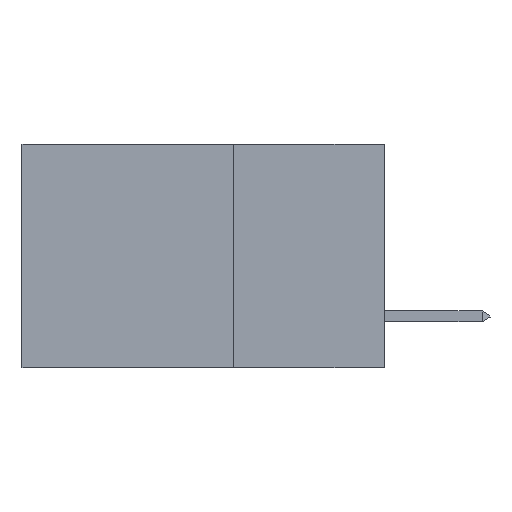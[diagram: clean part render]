
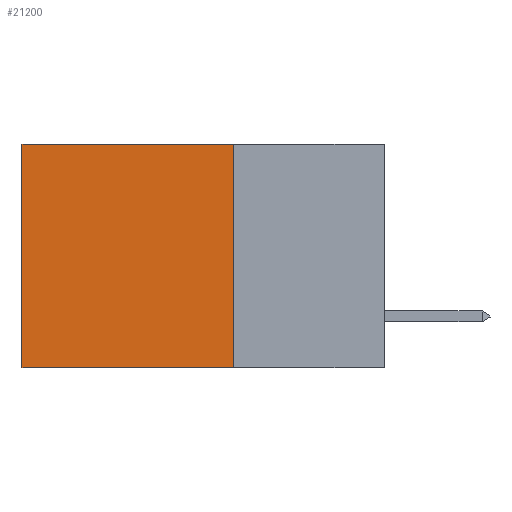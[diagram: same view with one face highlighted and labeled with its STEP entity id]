
A CAD part, left-side view. The second image highlights one B-rep face of the part: STEP entity #21200.
In plain terms, the highlighted planar face has unit normal (-1, 0, 0).
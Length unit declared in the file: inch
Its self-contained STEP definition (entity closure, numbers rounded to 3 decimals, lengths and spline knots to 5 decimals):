
#949 = FACE_OUTER_BOUND ( 'NONE', #18222, .T. ) ;
#1046 = VERTEX_POINT ( 'NONE', #7739 ) ;
#1164 = AXIS2_PLACEMENT_3D ( 'NONE', #21474, #10607, #21871 ) ;
#1707 = DIRECTION ( 'NONE',  ( 0., 0., -1. ) ) ;
#2795 = DIRECTION ( 'NONE',  ( 0., 1., 0. ) ) ;
#3478 = DIRECTION ( 'NONE',  ( 0., 1., 0. ) ) ;
#4974 = EDGE_CURVE ( 'NONE', #7376, #13451, #21937, .T. ) ;
#6647 = CARTESIAN_POINT ( 'NONE',  ( 0.2875, 0.6, 0. ) ) ;
#6938 = CARTESIAN_POINT ( 'NONE',  ( 0.2875, 0.25, -0.37 ) ) ;
#7376 = VERTEX_POINT ( 'NONE', #16361 ) ;
#7659 = LINE ( 'NONE', #6938, #8330 ) ;
#7739 = CARTESIAN_POINT ( 'NONE',  ( 0.2875, 0.6, -0.37 ) ) ;
#8107 = DIRECTION ( 'NONE',  ( 0., 0., -1. ) ) ;
#8330 = VECTOR ( 'NONE', #2795, 39.37008 ) ;
#8771 = VECTOR ( 'NONE', #3478, 39.37008 ) ;
#10059 = EDGE_CURVE ( 'NONE', #13451, #1046, #14945, .T. ) ;
#10607 = DIRECTION ( 'NONE',  ( 1., 0., 0. ) ) ;
#10647 = EDGE_CURVE ( 'NONE', #7376, #24971, #27778, .T. ) ;
#11084 = ORIENTED_EDGE ( 'NONE', *, *, #10647, .F. ) ;
#12670 = CARTESIAN_POINT ( 'NONE',  ( 0.2875, 0.6, 0. ) ) ;
#13451 = VERTEX_POINT ( 'NONE', #6647 ) ;
#14312 = CARTESIAN_POINT ( 'NONE',  ( 0.2875, 0.25, 0. ) ) ;
#14598 = CARTESIAN_POINT ( 'NONE',  ( 0.2875, 0.25, -0.37 ) ) ;
#14945 = LINE ( 'NONE', #12670, #28131 ) ;
#16361 = CARTESIAN_POINT ( 'NONE',  ( 0.2875, 0.25, 0. ) ) ;
#16675 = ORIENTED_EDGE ( 'NONE', *, *, #23348, .F. ) ;
#18222 = EDGE_LOOP ( 'NONE', ( #27862, #16675, #11084, #28127 ) ) ;
#21200 = ADVANCED_FACE ( 'NONE', ( #949 ), #28425, .F. ) ;
#21474 = CARTESIAN_POINT ( 'NONE',  ( 0.2875, 0.25, 0. ) ) ;
#21871 = DIRECTION ( 'NONE',  ( 0., 0., -1. ) ) ;
#21927 = VECTOR ( 'NONE', #8107, 39.37008 ) ;
#21937 = LINE ( 'NONE', #14312, #8771 ) ;
#23348 = EDGE_CURVE ( 'NONE', #24971, #1046, #7659, .T. ) ;
#24971 = VERTEX_POINT ( 'NONE', #14598 ) ;
#25709 = CARTESIAN_POINT ( 'NONE',  ( 0.2875, 0.25, 0. ) ) ;
#27778 = LINE ( 'NONE', #25709, #21927 ) ;
#27862 = ORIENTED_EDGE ( 'NONE', *, *, #10059, .T. ) ;
#28127 = ORIENTED_EDGE ( 'NONE', *, *, #4974, .T. ) ;
#28131 = VECTOR ( 'NONE', #1707, 39.37008 ) ;
#28425 = PLANE ( 'NONE',  #1164 ) ;
